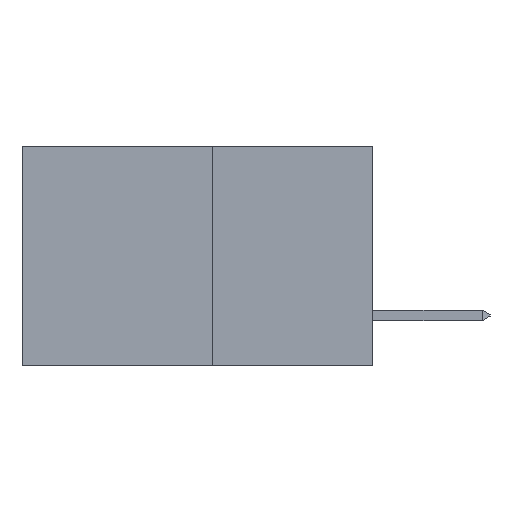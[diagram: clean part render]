
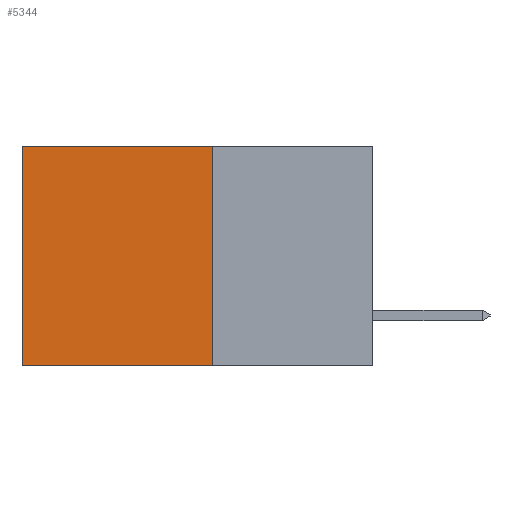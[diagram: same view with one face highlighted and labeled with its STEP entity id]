
A CAD part, left-side view. The second image highlights one B-rep face of the part: STEP entity #5344.
In plain terms, the highlighted planar face has unit normal (-1, 0, 0).
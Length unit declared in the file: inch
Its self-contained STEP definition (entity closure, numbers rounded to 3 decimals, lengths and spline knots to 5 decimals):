
#5344 = ADVANCED_FACE ( 'NONE', ( #32359 ), #15968, .F. ) ;
#5928 = DIRECTION ( 'NONE',  ( 0., 0., -1. ) ) ;
#5994 = EDGE_CURVE ( 'NONE', #21656, #20746, #19827, .T. ) ;
#7147 = CARTESIAN_POINT ( 'NONE',  ( 0.277, 0.27, -0.37 ) ) ;
#9509 = CARTESIAN_POINT ( 'NONE',  ( 0.277, 0.27, 0. ) ) ;
#13705 = VERTEX_POINT ( 'NONE', #31720 ) ;
#13713 = VECTOR ( 'NONE', #22728, 39.37008 ) ;
#14052 = VECTOR ( 'NONE', #30874, 39.37008 ) ;
#14372 = CARTESIAN_POINT ( 'NONE',  ( 0.277, 0.27, -0.37 ) ) ;
#14634 = VERTEX_POINT ( 'NONE', #9509 ) ;
#14810 = EDGE_CURVE ( 'NONE', #14634, #13705, #27791, .T. ) ;
#15257 = LINE ( 'NONE', #16224, #27389 ) ;
#15405 = CARTESIAN_POINT ( 'NONE',  ( 0.277, 0.27, 0. ) ) ;
#15888 = CARTESIAN_POINT ( 'NONE',  ( 0.277, 0.27, -0.37 ) ) ;
#15968 = PLANE ( 'NONE',  #24800 ) ;
#16224 = CARTESIAN_POINT ( 'NONE',  ( 0.277, 0.59, -0.37 ) ) ;
#18229 = ORIENTED_EDGE ( 'NONE', *, *, #19900, .F. ) ;
#18859 = ORIENTED_EDGE ( 'NONE', *, *, #28751, .T. ) ;
#19437 = ORIENTED_EDGE ( 'NONE', *, *, #14810, .T. ) ;
#19827 = LINE ( 'NONE', #26719, #24324 ) ;
#19900 = EDGE_CURVE ( 'NONE', #14634, #21656, #20577, .T. ) ;
#20325 = DIRECTION ( 'NONE',  ( 1., 0., 0. ) ) ;
#20577 = LINE ( 'NONE', #7147, #13713 ) ;
#20746 = VERTEX_POINT ( 'NONE', #23846 ) ;
#21656 = VERTEX_POINT ( 'NONE', #14372 ) ;
#22728 = DIRECTION ( 'NONE',  ( 0., 0., -1. ) ) ;
#23078 = DIRECTION ( 'NONE',  ( 0., 0., -1. ) ) ;
#23846 = CARTESIAN_POINT ( 'NONE',  ( 0.277, 0.59, -0.37 ) ) ;
#24324 = VECTOR ( 'NONE', #26095, 39.37008 ) ;
#24800 = AXIS2_PLACEMENT_3D ( 'NONE', #15888, #20325, #23078 ) ;
#26095 = DIRECTION ( 'NONE',  ( 0., 1., 0. ) ) ;
#26719 = CARTESIAN_POINT ( 'NONE',  ( 0.277, 0.27, -0.37 ) ) ;
#27389 = VECTOR ( 'NONE', #5928, 39.37008 ) ;
#27791 = LINE ( 'NONE', #15405, #14052 ) ;
#28179 = EDGE_LOOP ( 'NONE', ( #18859, #32454, #18229, #19437 ) ) ;
#28751 = EDGE_CURVE ( 'NONE', #13705, #20746, #15257, .T. ) ;
#30874 = DIRECTION ( 'NONE',  ( 0., 1., 0. ) ) ;
#31720 = CARTESIAN_POINT ( 'NONE',  ( 0.277, 0.59, 0. ) ) ;
#32359 = FACE_OUTER_BOUND ( 'NONE', #28179, .T. ) ;
#32454 = ORIENTED_EDGE ( 'NONE', *, *, #5994, .F. ) ;
